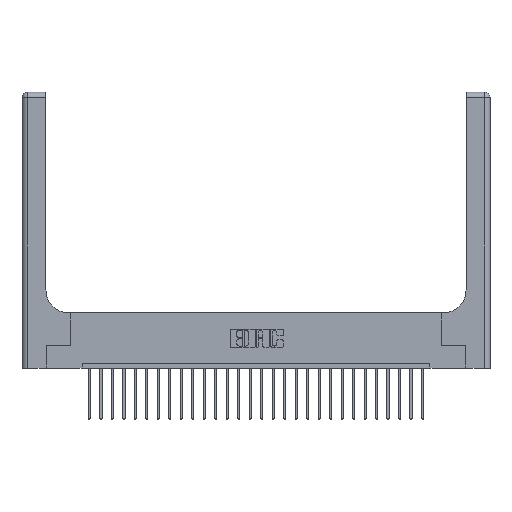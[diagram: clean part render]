
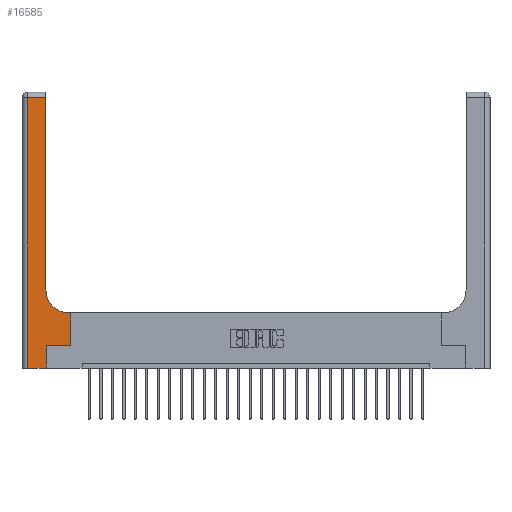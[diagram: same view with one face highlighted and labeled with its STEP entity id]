
A CAD part, top view. The second image highlights one B-rep face of the part: STEP entity #16585.
In plain terms, the highlighted planar face has unit normal (0, 0, 1).
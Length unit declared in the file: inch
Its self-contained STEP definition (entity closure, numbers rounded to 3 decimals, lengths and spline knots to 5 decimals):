
#139 = ORIENTED_EDGE ( 'NONE', *, *, #12275, .T. ) ;
#409 = AXIS2_PLACEMENT_3D ( 'NONE', #23350, #21384, #11554 ) ;
#1097 = CARTESIAN_POINT ( 'NONE',  ( 0.265, 0.25, 0.37 ) ) ;
#1281 = ORIENTED_EDGE ( 'NONE', *, *, #18478, .T. ) ;
#1452 = ORIENTED_EDGE ( 'NONE', *, *, #16898, .T. ) ;
#1704 = FACE_OUTER_BOUND ( 'NONE', #24081, .T. ) ;
#1991 = ORIENTED_EDGE ( 'NONE', *, *, #4570, .T. ) ;
#2571 = CIRCLE ( 'NONE', #409, 0.25 ) ;
#2616 = VECTOR ( 'NONE', #10446, 39.37008 ) ;
#2696 = CARTESIAN_POINT ( 'NONE',  ( 0.06, 0., 0.37 ) ) ;
#2835 = DIRECTION ( 'NONE',  ( 0., 1., 0. ) ) ;
#2840 = CARTESIAN_POINT ( 'NONE',  ( 0.26, 2.94, 0.37 ) ) ;
#2902 = DIRECTION ( 'NONE',  ( -1., 0., 0. ) ) ;
#3133 = PLANE ( 'NONE',  #15850 ) ;
#3152 = DIRECTION ( 'NONE',  ( 1., 0., 0. ) ) ;
#3688 = VECTOR ( 'NONE', #23170, 39.37008 ) ;
#4454 = ORIENTED_EDGE ( 'NONE', *, *, #11285, .T. ) ;
#4570 = EDGE_CURVE ( 'NONE', #20955, #12892, #23257, .T. ) ;
#5504 = DIRECTION ( 'NONE',  ( -1., 0., 0. ) ) ;
#5694 = CARTESIAN_POINT ( 'NONE',  ( 0.26, 3., 0.37 ) ) ;
#5928 = LINE ( 'NONE', #13505, #10563 ) ;
#6167 = CARTESIAN_POINT ( 'NONE',  ( 0.51, 0.6, 0.37 ) ) ;
#6526 = VERTEX_POINT ( 'NONE', #13739 ) ;
#6809 = VERTEX_POINT ( 'NONE', #2840 ) ;
#6872 = VECTOR ( 'NONE', #2902, 39.37008 ) ;
#6873 = CARTESIAN_POINT ( 'NONE',  ( 0., 0., 0.37 ) ) ;
#7260 = VERTEX_POINT ( 'NONE', #17098 ) ;
#9094 = VECTOR ( 'NONE', #11264, 39.37008 ) ;
#9473 = CARTESIAN_POINT ( 'NONE',  ( 0.26, 0.6, 0.37 ) ) ;
#9515 = VERTEX_POINT ( 'NONE', #6167 ) ;
#10446 = DIRECTION ( 'NONE',  ( 0., 1., 0. ) ) ;
#10563 = VECTOR ( 'NONE', #13585, 39.37008 ) ;
#10635 = LINE ( 'NONE', #24277, #18338 ) ;
#10880 = VERTEX_POINT ( 'NONE', #16242 ) ;
#11184 = LINE ( 'NONE', #18771, #6872 ) ;
#11247 = LINE ( 'NONE', #20611, #2616 ) ;
#11264 = DIRECTION ( 'NONE',  ( 1., 0., 0. ) ) ;
#11285 = EDGE_CURVE ( 'NONE', #9515, #19428, #2571, .T. ) ;
#11438 = CARTESIAN_POINT ( 'NONE',  ( 0.265, 0.25, 0.37 ) ) ;
#11554 = DIRECTION ( 'NONE',  ( 1., 0., 0. ) ) ;
#12275 = EDGE_CURVE ( 'NONE', #6809, #10880, #11184, .T. ) ;
#12892 = VERTEX_POINT ( 'NONE', #19442 ) ;
#12899 = DIRECTION ( 'NONE',  ( 0., 0., -1. ) ) ;
#13505 = CARTESIAN_POINT ( 'NONE',  ( 0.06, 3., 0.37 ) ) ;
#13585 = DIRECTION ( 'NONE',  ( 0., -1., 0. ) ) ;
#13739 = CARTESIAN_POINT ( 'NONE',  ( 0.265, 0., 0.37 ) ) ;
#14494 = ORIENTED_EDGE ( 'NONE', *, *, #19559, .T. ) ;
#14547 = VECTOR ( 'NONE', #5504, 39.37008 ) ;
#14798 = LINE ( 'NONE', #5694, #3688 ) ;
#15407 = ORIENTED_EDGE ( 'NONE', *, *, #21442, .T. ) ;
#15850 = AXIS2_PLACEMENT_3D ( 'NONE', #20544, #12899, #16943 ) ;
#16242 = CARTESIAN_POINT ( 'NONE',  ( 0.06, 2.94, 0.37 ) ) ;
#16585 = ADVANCED_FACE ( 'NONE', ( #1704 ), #3133, .F. ) ;
#16898 = EDGE_CURVE ( 'NONE', #12892, #7260, #11247, .T. ) ;
#16943 = DIRECTION ( 'NONE',  ( -1., 0., 0. ) ) ;
#17098 = CARTESIAN_POINT ( 'NONE',  ( 0.528, 0.6, 0.37 ) ) ;
#17878 = CARTESIAN_POINT ( 'NONE',  ( 0.26, 0.85, 0.37 ) ) ;
#18329 = EDGE_CURVE ( 'NONE', #7260, #9515, #23507, .T. ) ;
#18338 = VECTOR ( 'NONE', #2835, 39.37008 ) ;
#18478 = EDGE_CURVE ( 'NONE', #10880, #23919, #5928, .T. ) ;
#18771 = CARTESIAN_POINT ( 'NONE',  ( 0., 2.94, 0.37 ) ) ;
#19393 = ORIENTED_EDGE ( 'NONE', *, *, #18329, .T. ) ;
#19428 = VERTEX_POINT ( 'NONE', #17878 ) ;
#19442 = CARTESIAN_POINT ( 'NONE',  ( 0.528, 0.25, 0.37 ) ) ;
#19559 = EDGE_CURVE ( 'NONE', #23919, #6526, #21328, .T. ) ;
#20544 = CARTESIAN_POINT ( 'NONE',  ( 0., 3., 0.37 ) ) ;
#20611 = CARTESIAN_POINT ( 'NONE',  ( 0.528, 0.25, 0.37 ) ) ;
#20620 = EDGE_CURVE ( 'NONE', #19428, #6809, #14798, .T. ) ;
#20955 = VERTEX_POINT ( 'NONE', #1097 ) ;
#21328 = LINE ( 'NONE', #6873, #22837 ) ;
#21384 = DIRECTION ( 'NONE',  ( 0., 0., -1. ) ) ;
#21442 = EDGE_CURVE ( 'NONE', #6526, #20955, #10635, .T. ) ;
#22068 = ORIENTED_EDGE ( 'NONE', *, *, #20620, .T. ) ;
#22837 = VECTOR ( 'NONE', #3152, 39.37008 ) ;
#23170 = DIRECTION ( 'NONE',  ( 0., 1., 0. ) ) ;
#23257 = LINE ( 'NONE', #11438, #9094 ) ;
#23350 = CARTESIAN_POINT ( 'NONE',  ( 0.51, 0.85, 0.37 ) ) ;
#23507 = LINE ( 'NONE', #9473, #14547 ) ;
#23919 = VERTEX_POINT ( 'NONE', #2696 ) ;
#24081 = EDGE_LOOP ( 'NONE', ( #22068, #139, #1281, #14494, #15407, #1991, #1452, #19393, #4454 ) ) ;
#24277 = CARTESIAN_POINT ( 'NONE',  ( 0.265, 0., 0.37 ) ) ;
